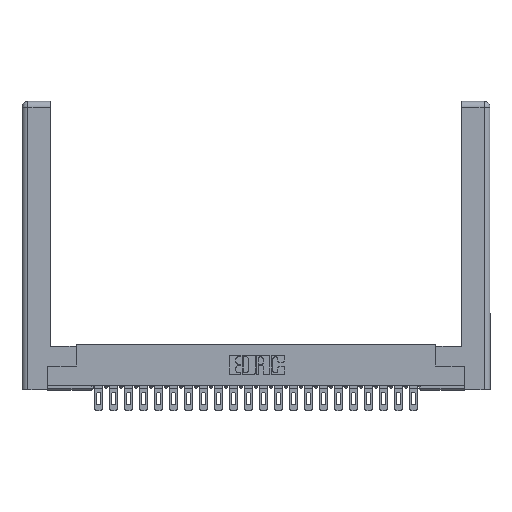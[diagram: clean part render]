
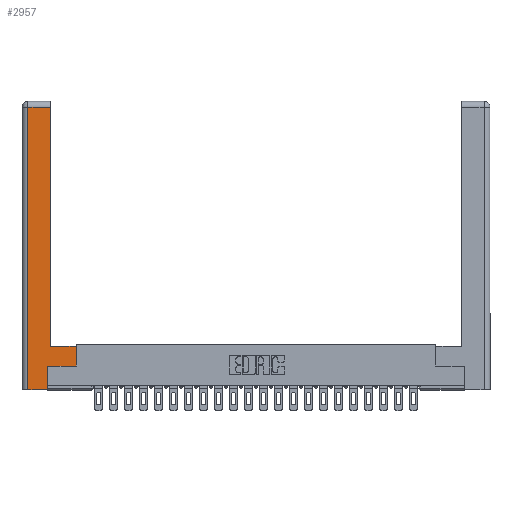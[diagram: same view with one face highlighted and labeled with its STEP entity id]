
A CAD part, top view. The second image highlights one B-rep face of the part: STEP entity #2957.
In plain terms, the highlighted planar face has unit normal (0, 0, 1).
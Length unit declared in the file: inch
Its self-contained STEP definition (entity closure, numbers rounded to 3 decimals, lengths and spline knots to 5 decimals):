
#22 = CARTESIAN_POINT ( 'NONE',  ( 0.265, 0.245, 0. ) ) ;
#325 = ORIENTED_EDGE ( 'NONE', *, *, #21730, .T. ) ;
#551 = AXIS2_PLACEMENT_3D ( 'NONE', #23666, #6515, #14145 ) ;
#1125 = LINE ( 'NONE', #16645, #8697 ) ;
#2957 = ADVANCED_FACE ( 'NONE', ( #16020 ), #6628, .F. ) ;
#3636 = VERTEX_POINT ( 'NONE', #10465 ) ;
#4603 = CARTESIAN_POINT ( 'NONE',  ( 0.295, 0.45, 0. ) ) ;
#4983 = LINE ( 'NONE', #16239, #20866 ) ;
#5035 = CARTESIAN_POINT ( 'NONE',  ( 0.0615, 2.94, 0. ) ) ;
#5083 = LINE ( 'NONE', #9086, #13965 ) ;
#5098 = EDGE_CURVE ( 'NONE', #16052, #3636, #12709, .T. ) ;
#5409 = VERTEX_POINT ( 'NONE', #10314 ) ;
#6515 = DIRECTION ( 'NONE',  ( 0., 0., -1. ) ) ;
#6567 = VERTEX_POINT ( 'NONE', #12088 ) ;
#6628 = PLANE ( 'NONE',  #551 ) ;
#6700 = CARTESIAN_POINT ( 'NONE',  ( 0.0615, 0., 0. ) ) ;
#7076 = ORIENTED_EDGE ( 'NONE', *, *, #24530, .T. ) ;
#7404 = CARTESIAN_POINT ( 'NONE',  ( 0.565, 0.245, 0. ) ) ;
#7797 = LINE ( 'NONE', #22, #9540 ) ;
#8502 = VECTOR ( 'NONE', #15338, 39.37008 ) ;
#8697 = VECTOR ( 'NONE', #13030, 39.37008 ) ;
#8786 = DIRECTION ( 'NONE',  ( 0., 1., 0. ) ) ;
#8884 = VERTEX_POINT ( 'NONE', #5035 ) ;
#9086 = CARTESIAN_POINT ( 'NONE',  ( 0.295, 0.45, 0. ) ) ;
#9147 = DIRECTION ( 'NONE',  ( 1., 0., 0. ) ) ;
#9329 = CARTESIAN_POINT ( 'NONE',  ( 0.0615, 2.94, 0. ) ) ;
#9540 = VECTOR ( 'NONE', #13316, 39.37008 ) ;
#9721 = EDGE_CURVE ( 'NONE', #8884, #14772, #4983, .T. ) ;
#10180 = EDGE_CURVE ( 'NONE', #24168, #8884, #18966, .T. ) ;
#10314 = CARTESIAN_POINT ( 'NONE',  ( 0.265, 0., 0. ) ) ;
#10465 = CARTESIAN_POINT ( 'NONE',  ( 0.565, 0.45, 0. ) ) ;
#11722 = ORIENTED_EDGE ( 'NONE', *, *, #9721, .T. ) ;
#12088 = CARTESIAN_POINT ( 'NONE',  ( 0.265, 0.245, 0. ) ) ;
#12195 = ORIENTED_EDGE ( 'NONE', *, *, #12408, .T. ) ;
#12408 = EDGE_CURVE ( 'NONE', #15561, #24168, #18169, .T. ) ;
#12709 = LINE ( 'NONE', #22336, #21448 ) ;
#13030 = DIRECTION ( 'NONE',  ( 1., 0., 0. ) ) ;
#13057 = ORIENTED_EDGE ( 'NONE', *, *, #10180, .T. ) ;
#13316 = DIRECTION ( 'NONE',  ( 0., 1., 0. ) ) ;
#13965 = VECTOR ( 'NONE', #16718, 39.37008 ) ;
#14145 = DIRECTION ( 'NONE',  ( -1., 0., 0. ) ) ;
#14703 = DIRECTION ( 'NONE',  ( 0., 1., 0. ) ) ;
#14772 = VERTEX_POINT ( 'NONE', #6700 ) ;
#14960 = CARTESIAN_POINT ( 'NONE',  ( 0.565, 0.245, 0. ) ) ;
#15338 = DIRECTION ( 'NONE',  ( -1., 0., 0. ) ) ;
#15561 = VERTEX_POINT ( 'NONE', #4603 ) ;
#16020 = FACE_OUTER_BOUND ( 'NONE', #24193, .T. ) ;
#16052 = VERTEX_POINT ( 'NONE', #14960 ) ;
#16239 = CARTESIAN_POINT ( 'NONE',  ( 0.0615, 0., 0. ) ) ;
#16491 = DIRECTION ( 'NONE',  ( 0., -1., 0. ) ) ;
#16645 = CARTESIAN_POINT ( 'NONE',  ( 0.265, 0., 0. ) ) ;
#16718 = DIRECTION ( 'NONE',  ( -1., 0., 0. ) ) ;
#18169 = LINE ( 'NONE', #20173, #22050 ) ;
#18361 = EDGE_CURVE ( 'NONE', #14772, #5409, #1125, .T. ) ;
#18966 = LINE ( 'NONE', #9329, #8502 ) ;
#19072 = ORIENTED_EDGE ( 'NONE', *, *, #5098, .T. ) ;
#19357 = EDGE_CURVE ( 'NONE', #5409, #6567, #7797, .T. ) ;
#20173 = CARTESIAN_POINT ( 'NONE',  ( 0.295, 3., 0. ) ) ;
#20866 = VECTOR ( 'NONE', #16491, 39.37008 ) ;
#21384 = CARTESIAN_POINT ( 'NONE',  ( 0.295, 2.94, 0. ) ) ;
#21448 = VECTOR ( 'NONE', #14703, 39.37008 ) ;
#21730 = EDGE_CURVE ( 'NONE', #6567, #16052, #22175, .T. ) ;
#22050 = VECTOR ( 'NONE', #8786, 39.37008 ) ;
#22175 = LINE ( 'NONE', #7404, #24432 ) ;
#22336 = CARTESIAN_POINT ( 'NONE',  ( 0.565, 0.45, 0. ) ) ;
#23666 = CARTESIAN_POINT ( 'NONE',  ( 0., 0., 0. ) ) ;
#24168 = VERTEX_POINT ( 'NONE', #21384 ) ;
#24185 = ORIENTED_EDGE ( 'NONE', *, *, #19357, .T. ) ;
#24193 = EDGE_LOOP ( 'NONE', ( #12195, #13057, #11722, #24353, #24185, #325, #19072, #7076 ) ) ;
#24353 = ORIENTED_EDGE ( 'NONE', *, *, #18361, .T. ) ;
#24432 = VECTOR ( 'NONE', #9147, 39.37008 ) ;
#24530 = EDGE_CURVE ( 'NONE', #3636, #15561, #5083, .T. ) ;
